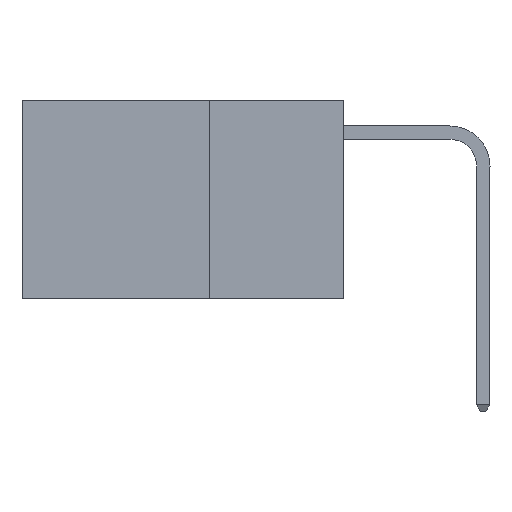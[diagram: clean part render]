
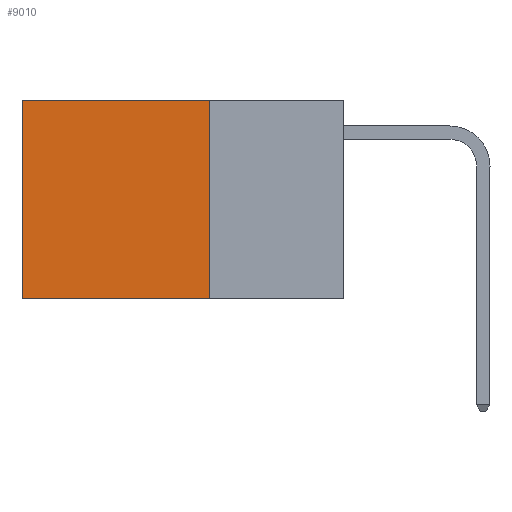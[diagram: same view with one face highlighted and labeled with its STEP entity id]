
A CAD part, left-side view. The second image highlights one B-rep face of the part: STEP entity #9010.
In plain terms, the highlighted planar face has unit normal (-1, 0, 0).
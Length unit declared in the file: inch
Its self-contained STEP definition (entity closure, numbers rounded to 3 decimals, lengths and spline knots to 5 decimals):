
#165 = CARTESIAN_POINT ( 'NONE',  ( 0.2625, 0.25, 0. ) ) ;
#1662 = DIRECTION ( 'NONE',  ( 0., 0., -1. ) ) ;
#2132 = VERTEX_POINT ( 'NONE', #8336 ) ;
#2558 = VECTOR ( 'NONE', #14134, 39.37008 ) ;
#3143 = VERTEX_POINT ( 'NONE', #6409 ) ;
#3588 = DIRECTION ( 'NONE',  ( 0., 1., 0. ) ) ;
#3681 = ORIENTED_EDGE ( 'NONE', *, *, #13701, .F. ) ;
#3899 = VECTOR ( 'NONE', #10842, 39.37008 ) ;
#4558 = CARTESIAN_POINT ( 'NONE',  ( 0.2625, 0.25, 0. ) ) ;
#4719 = VECTOR ( 'NONE', #1662, 39.37008 ) ;
#5550 = ORIENTED_EDGE ( 'NONE', *, *, #18313, .F. ) ;
#5998 = ORIENTED_EDGE ( 'NONE', *, *, #9595, .T. ) ;
#6243 = FACE_OUTER_BOUND ( 'NONE', #11960, .T. ) ;
#6409 = CARTESIAN_POINT ( 'NONE',  ( 0.2625, 0.6, 0. ) ) ;
#6964 = LINE ( 'NONE', #8342, #2558 ) ;
#8336 = CARTESIAN_POINT ( 'NONE',  ( 0.2625, 0.6, -0.37 ) ) ;
#8342 = CARTESIAN_POINT ( 'NONE',  ( 0.2625, 0.25, 0. ) ) ;
#9010 = ADVANCED_FACE ( 'NONE', ( #6243 ), #14912, .F. ) ;
#9096 = DIRECTION ( 'NONE',  ( 0., 0., -1. ) ) ;
#9595 = EDGE_CURVE ( 'NONE', #3143, #2132, #12217, .T. ) ;
#10109 = CARTESIAN_POINT ( 'NONE',  ( 0.2625, 0.25, 0. ) ) ;
#10761 = VECTOR ( 'NONE', #3588, 39.37008 ) ;
#10842 = DIRECTION ( 'NONE',  ( 0., 0., -1. ) ) ;
#11960 = EDGE_LOOP ( 'NONE', ( #5998, #3681, #5550, #11992 ) ) ;
#11992 = ORIENTED_EDGE ( 'NONE', *, *, #16274, .T. ) ;
#12217 = LINE ( 'NONE', #18115, #3899 ) ;
#13701 = EDGE_CURVE ( 'NONE', #18332, #2132, #18514, .T. ) ;
#14068 = AXIS2_PLACEMENT_3D ( 'NONE', #4558, #17857, #9096 ) ;
#14134 = DIRECTION ( 'NONE',  ( 0., 1., 0. ) ) ;
#14912 = PLANE ( 'NONE',  #14068 ) ;
#15375 = CARTESIAN_POINT ( 'NONE',  ( 0.2625, 0.25, -0.37 ) ) ;
#15537 = LINE ( 'NONE', #165, #4719 ) ;
#16274 = EDGE_CURVE ( 'NONE', #17770, #3143, #6964, .T. ) ;
#16430 = CARTESIAN_POINT ( 'NONE',  ( 0.2625, 0.25, -0.37 ) ) ;
#17770 = VERTEX_POINT ( 'NONE', #10109 ) ;
#17857 = DIRECTION ( 'NONE',  ( 1., 0., 0. ) ) ;
#18115 = CARTESIAN_POINT ( 'NONE',  ( 0.2625, 0.6, 0. ) ) ;
#18313 = EDGE_CURVE ( 'NONE', #17770, #18332, #15537, .T. ) ;
#18332 = VERTEX_POINT ( 'NONE', #16430 ) ;
#18514 = LINE ( 'NONE', #15375, #10761 ) ;
